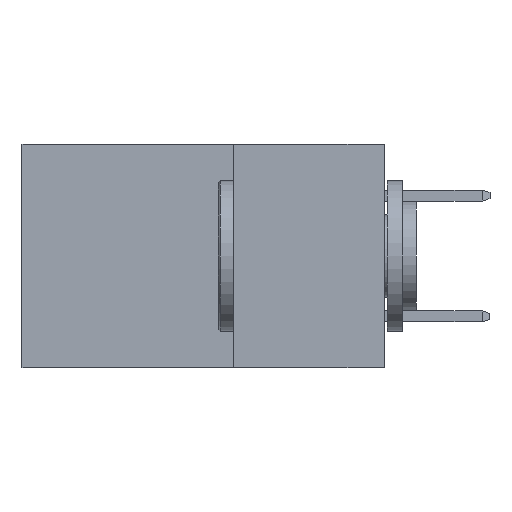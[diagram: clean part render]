
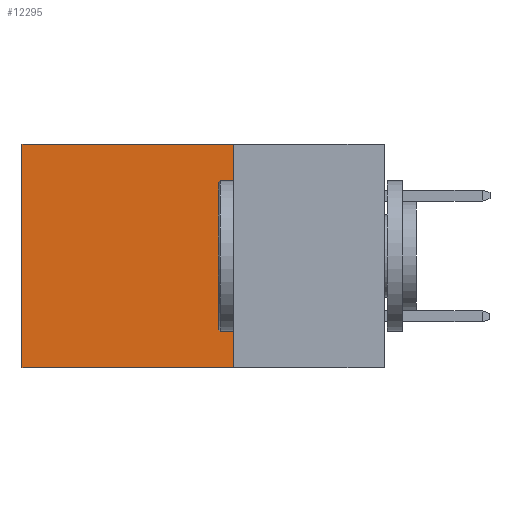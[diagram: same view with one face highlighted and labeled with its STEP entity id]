
A CAD part, left-side view. The second image highlights one B-rep face of the part: STEP entity #12295.
In plain terms, the highlighted planar face has unit normal (-1, 0, 0).
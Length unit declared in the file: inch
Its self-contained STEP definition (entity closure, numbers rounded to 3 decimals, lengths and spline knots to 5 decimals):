
#247 = VECTOR ( 'NONE', #13782, 39.37008 ) ;
#346 = EDGE_CURVE ( 'NONE', #5893, #13908, #8541, .T. ) ;
#536 = CARTESIAN_POINT ( 'NONE',  ( 0.298, 0.25, -0.37 ) ) ;
#2147 = VECTOR ( 'NONE', #13923, 39.37008 ) ;
#2909 = LINE ( 'NONE', #4770, #247 ) ;
#3604 = CARTESIAN_POINT ( 'NONE',  ( 0.298, 0.6, 0. ) ) ;
#3827 = CARTESIAN_POINT ( 'NONE',  ( 0.298, 0.25, 0. ) ) ;
#3917 = VERTEX_POINT ( 'NONE', #12419 ) ;
#4274 = CARTESIAN_POINT ( 'NONE',  ( 0.298, 0.6, 0. ) ) ;
#4322 = CARTESIAN_POINT ( 'NONE',  ( 0.298, 0.25, -0.37 ) ) ;
#4770 = CARTESIAN_POINT ( 'NONE',  ( 0.298, 0.25, 0. ) ) ;
#5111 = VECTOR ( 'NONE', #14716, 39.37008 ) ;
#5120 = DIRECTION ( 'NONE',  ( 0., 0., -1. ) ) ;
#5603 = DIRECTION ( 'NONE',  ( 0., 1., 0. ) ) ;
#5893 = VERTEX_POINT ( 'NONE', #9513 ) ;
#6183 = FACE_OUTER_BOUND ( 'NONE', #6640, .T. ) ;
#6263 = LINE ( 'NONE', #4322, #16008 ) ;
#6640 = EDGE_LOOP ( 'NONE', ( #7569, #7621, #10459, #10191 ) ) ;
#7569 = ORIENTED_EDGE ( 'NONE', *, *, #13458, .T. ) ;
#7621 = ORIENTED_EDGE ( 'NONE', *, *, #14688, .F. ) ;
#8541 = LINE ( 'NONE', #14838, #5111 ) ;
#9037 = VERTEX_POINT ( 'NONE', #4274 ) ;
#9147 = EDGE_CURVE ( 'NONE', #5893, #9037, #2909, .T. ) ;
#9513 = CARTESIAN_POINT ( 'NONE',  ( 0.298, 0.25, 0. ) ) ;
#10191 = ORIENTED_EDGE ( 'NONE', *, *, #9147, .T. ) ;
#10459 = ORIENTED_EDGE ( 'NONE', *, *, #346, .F. ) ;
#11502 = PLANE ( 'NONE',  #15298 ) ;
#12295 = ADVANCED_FACE ( 'NONE', ( #6183 ), #11502, .F. ) ;
#12419 = CARTESIAN_POINT ( 'NONE',  ( 0.298, 0.6, -0.37 ) ) ;
#12446 = LINE ( 'NONE', #3604, #2147 ) ;
#12848 = DIRECTION ( 'NONE',  ( 1., 0., 0. ) ) ;
#13458 = EDGE_CURVE ( 'NONE', #9037, #3917, #12446, .T. ) ;
#13782 = DIRECTION ( 'NONE',  ( 0., 1., 0. ) ) ;
#13908 = VERTEX_POINT ( 'NONE', #536 ) ;
#13923 = DIRECTION ( 'NONE',  ( 0., 0., -1. ) ) ;
#14688 = EDGE_CURVE ( 'NONE', #13908, #3917, #6263, .T. ) ;
#14716 = DIRECTION ( 'NONE',  ( 0., 0., -1. ) ) ;
#14838 = CARTESIAN_POINT ( 'NONE',  ( 0.298, 0.25, 0. ) ) ;
#15298 = AXIS2_PLACEMENT_3D ( 'NONE', #3827, #12848, #5120 ) ;
#16008 = VECTOR ( 'NONE', #5603, 39.37008 ) ;
